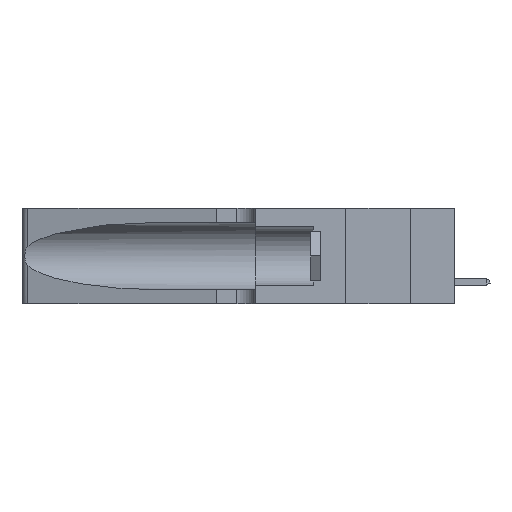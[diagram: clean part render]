
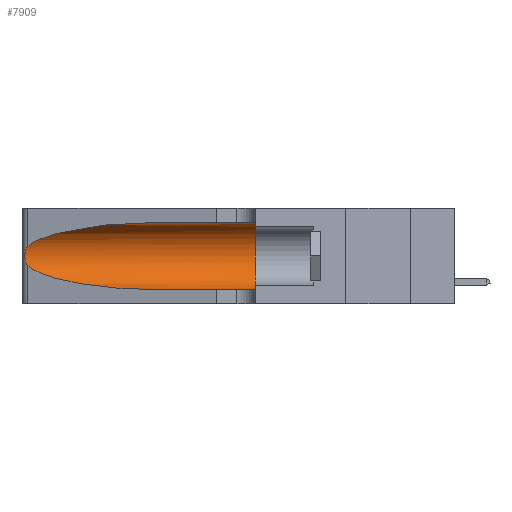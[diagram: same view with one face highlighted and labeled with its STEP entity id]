
A CAD part, left-side view. The second image highlights one B-rep face of the part: STEP entity #7909.
In plain terms, the highlighted cylindrical face has radius 3.308 mm (diameter 6.617 mm), a partial arc.
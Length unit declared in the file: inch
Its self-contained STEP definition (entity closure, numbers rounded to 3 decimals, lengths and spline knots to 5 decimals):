
#151 = ORIENTED_EDGE ( 'NONE', *, *, #31552, .F. ) ;
#303 = ORIENTED_EDGE ( 'NONE', *, *, #20251, .T. ) ;
#431 = CARTESIAN_POINT ( 'NONE',  ( 0.25789, 1.23486, 0.15765 ) ) ;
#638 = VECTOR ( 'NONE', #11944, 39.37008 ) ;
#2279 = EDGE_CURVE ( 'NONE', #34052, #12457, #35479, .T. ) ;
#2406 = CARTESIAN_POINT ( 'NONE',  ( 0.1305, 0.35, 0.05475 ) ) ;
#2992 = ORIENTED_EDGE ( 'NONE', *, *, #8890, .F. ) ;
#4071 = CARTESIAN_POINT ( 'NONE',  ( 0.1305, 0.72297, 0.31525 ) ) ;
#4332 = CARTESIAN_POINT ( 'NONE',  ( 0.18966, 0.96281, 0.31525 ) ) ;
#5220 =( BOUNDED_CURVE ( )  B_SPLINE_CURVE ( 3, ( #4071, #4332, #36761, #36890 ),
 .UNSPECIFIED., .F., .F. ) 
 B_SPLINE_CURVE_WITH_KNOTS ( ( 4, 4 ),
 ( 1.5708, 2.84003 ),
 .UNSPECIFIED. ) 
 CURVE ( )  GEOMETRIC_REPRESENTATION_ITEM ( )  RATIONAL_B_SPLINE_CURVE ( ( 1., 0.87, 0.87, 1. ) ) 
 REPRESENTATION_ITEM ( '' )  );
#5604 = CARTESIAN_POINT ( 'NONE',  ( 0.18966, 0.96281, 0.05475 ) ) ;
#5620 = DIRECTION ( 'NONE',  ( 0., -1., 0. ) ) ;
#7909 = ADVANCED_FACE ( 'NONE', ( #20787 ), #12911, .F. ) ;
#8056 = LINE ( 'NONE', #35334, #638 ) ;
#8890 = EDGE_CURVE ( 'NONE', #32274, #33741, #25790, .T. ) ;
#9158 = B_SPLINE_CURVE_WITH_KNOTS ( 'NONE', 3,
 ( #18841, #36635, #10705, #37280, #37543, #29770, #24171, #24298, #9587, #15837, #431, #19338, #27800, #27672 ),
 .UNSPECIFIED., .F., .F.,
 ( 4, 2, 2, 2, 2, 2, 4 ),
 ( 0., 0.00027, 0.00053, 0.00107, 0.0016, 0.00187, 0.00214 ),
 .UNSPECIFIED. ) ;
#9587 = CARTESIAN_POINT ( 'NONE',  ( 0.26017, 1.23833, 0.17102 ) ) ;
#10518 = EDGE_LOOP ( 'NONE', ( #35236, #303, #33572, #17297, #151, #2992 ) ) ;
#10705 = CARTESIAN_POINT ( 'NONE',  ( 0.25639, 1.23184, 0.21858 ) ) ;
#11678 = DIRECTION ( 'NONE',  ( 0., 0., 1. ) ) ;
#11944 = DIRECTION ( 'NONE',  ( 0., -1., 0. ) ) ;
#12457 = VERTEX_POINT ( 'NONE', #30204 ) ;
#12668 = AXIS2_PLACEMENT_3D ( 'NONE', #17325, #5620, #36121 ) ;
#12911 = CYLINDRICAL_SURFACE ( 'NONE', #12668, 0.13025 ) ;
#13001 = CARTESIAN_POINT ( 'NONE',  ( 0.1305, 0.35, 0.31525 ) ) ;
#13473 = AXIS2_PLACEMENT_3D ( 'NONE', #17505, #14301, #11678 ) ;
#14301 = DIRECTION ( 'NONE',  ( 0., 1., 0. ) ) ;
#15041 = CARTESIAN_POINT ( 'NONE',  ( 0.25487, 1.22718, 0.14631 ) ) ;
#15837 = CARTESIAN_POINT ( 'NONE',  ( 0.25856, 1.23593, 0.16098 ) ) ;
#17297 = ORIENTED_EDGE ( 'NONE', *, *, #25300, .T. ) ;
#17325 = CARTESIAN_POINT ( 'NONE',  ( 0.1305, 1.61858, 0.185 ) ) ;
#17505 = CARTESIAN_POINT ( 'NONE',  ( 0.1305, 0.35, 0.185 ) ) ;
#18841 = CARTESIAN_POINT ( 'NONE',  ( 0.25487, 1.22718, 0.22369 ) ) ;
#19338 = CARTESIAN_POINT ( 'NONE',  ( 0.25639, 1.23186, 0.15144 ) ) ;
#20251 = EDGE_CURVE ( 'NONE', #37592, #34052, #9158, .T. ) ;
#20602 = VERTEX_POINT ( 'NONE', #2406 ) ;
#20787 = FACE_OUTER_BOUND ( 'NONE', #10518, .T. ) ;
#23021 = VECTOR ( 'NONE', #33426, 39.37008 ) ;
#23436 = CARTESIAN_POINT ( 'NONE',  ( 0.1305, 0.72297, 0.05475 ) ) ;
#23546 = CARTESIAN_POINT ( 'NONE',  ( 0.25487, 1.22718, 0.14631 ) ) ;
#24171 = CARTESIAN_POINT ( 'NONE',  ( 0.26075, 1.23896, 0.19203 ) ) ;
#24298 = CARTESIAN_POINT ( 'NONE',  ( 0.26075, 1.23896, 0.178 ) ) ;
#25300 = EDGE_CURVE ( 'NONE', #12457, #20602, #8056, .T. ) ;
#25790 = LINE ( 'NONE', #27486, #23021 ) ;
#27486 = CARTESIAN_POINT ( 'NONE',  ( 0.1305, 1.61858, 0.31525 ) ) ;
#27672 = CARTESIAN_POINT ( 'NONE',  ( 0.25487, 1.22718, 0.14631 ) ) ;
#27800 = CARTESIAN_POINT ( 'NONE',  ( 0.25555, 1.22993, 0.14849 ) ) ;
#29770 = CARTESIAN_POINT ( 'NONE',  ( 0.26018, 1.23835, 0.19895 ) ) ;
#30204 = CARTESIAN_POINT ( 'NONE',  ( 0.1305, 0.72297, 0.05475 ) ) ;
#30531 = EDGE_CURVE ( 'NONE', #32274, #37592, #5220, .T. ) ;
#31552 = EDGE_CURVE ( 'NONE', #33741, #20602, #36939, .T. ) ;
#32274 = VERTEX_POINT ( 'NONE', #33115 ) ;
#32344 = CARTESIAN_POINT ( 'NONE',  ( 0.2373, 1.15595, 0.08982 ) ) ;
#33115 = CARTESIAN_POINT ( 'NONE',  ( 0.1305, 0.72297, 0.31525 ) ) ;
#33426 = DIRECTION ( 'NONE',  ( 0., -1., 0. ) ) ;
#33572 = ORIENTED_EDGE ( 'NONE', *, *, #2279, .T. ) ;
#33741 = VERTEX_POINT ( 'NONE', #13001 ) ;
#33776 = CARTESIAN_POINT ( 'NONE',  ( 0.25487, 1.22718, 0.22369 ) ) ;
#34052 = VERTEX_POINT ( 'NONE', #15041 ) ;
#35236 = ORIENTED_EDGE ( 'NONE', *, *, #30531, .T. ) ;
#35334 = CARTESIAN_POINT ( 'NONE',  ( 0.1305, 1.61858, 0.05475 ) ) ;
#35479 =( BOUNDED_CURVE ( )  B_SPLINE_CURVE ( 3, ( #23546, #32344, #5604, #23436 ),
 .UNSPECIFIED., .F., .F. ) 
 B_SPLINE_CURVE_WITH_KNOTS ( ( 4, 4 ),
 ( 3.44316, 4.71239 ),
 .UNSPECIFIED. ) 
 CURVE ( )  GEOMETRIC_REPRESENTATION_ITEM ( )  RATIONAL_B_SPLINE_CURVE ( ( 1., 0.87, 0.87, 1. ) ) 
 REPRESENTATION_ITEM ( '' )  );
#36121 = DIRECTION ( 'NONE',  ( 0., 0., -1. ) ) ;
#36635 = CARTESIAN_POINT ( 'NONE',  ( 0.25555, 1.22994, 0.2215 ) ) ;
#36761 = CARTESIAN_POINT ( 'NONE',  ( 0.2373, 1.15595, 0.28018 ) ) ;
#36890 = CARTESIAN_POINT ( 'NONE',  ( 0.25487, 1.22718, 0.22369 ) ) ;
#36939 = CIRCLE ( 'NONE', #13473, 0.13025 ) ;
#37280 = CARTESIAN_POINT ( 'NONE',  ( 0.25787, 1.23484, 0.2124 ) ) ;
#37543 = CARTESIAN_POINT ( 'NONE',  ( 0.25854, 1.2359, 0.20912 ) ) ;
#37592 = VERTEX_POINT ( 'NONE', #33776 ) ;
